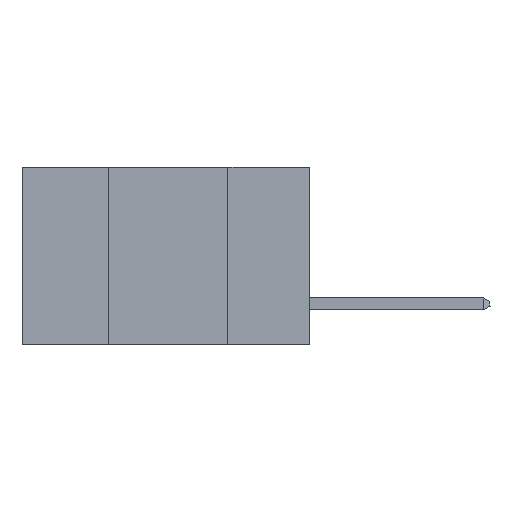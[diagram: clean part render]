
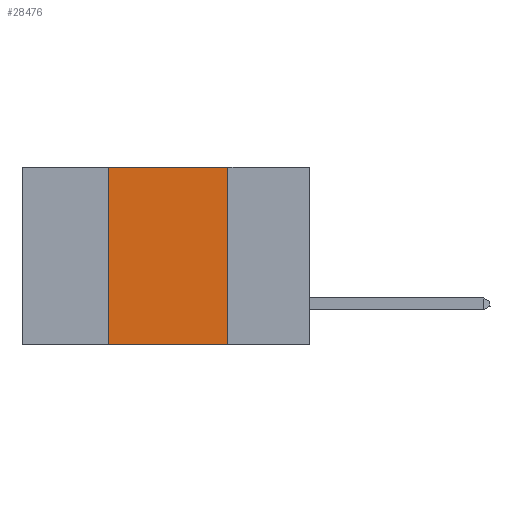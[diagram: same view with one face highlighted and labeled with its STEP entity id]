
A CAD part, left-side view. The second image highlights one B-rep face of the part: STEP entity #28476.
In plain terms, the highlighted planar face has unit normal (-1, 0, 0).
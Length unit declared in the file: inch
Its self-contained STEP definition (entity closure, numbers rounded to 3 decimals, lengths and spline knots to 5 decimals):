
#44 = CARTESIAN_POINT ( 'NONE',  ( 0., 0.6, 0. ) ) ;
#2948 = ORIENTED_EDGE ( 'NONE', *, *, #10224, .F. ) ;
#3013 = VERTEX_POINT ( 'NONE', #19193 ) ;
#5655 = CARTESIAN_POINT ( 'NONE',  ( 0., 0.42, -0.37 ) ) ;
#6412 = ORIENTED_EDGE ( 'NONE', *, *, #18906, .F. ) ;
#6725 = ORIENTED_EDGE ( 'NONE', *, *, #29199, .F. ) ;
#7812 = DIRECTION ( 'NONE',  ( 0., -1., 0. ) ) ;
#8812 = VECTOR ( 'NONE', #7812, 39.37008 ) ;
#9528 = DIRECTION ( 'NONE',  ( 0., 0., -1. ) ) ;
#9575 = DIRECTION ( 'NONE',  ( 1., 0., 0. ) ) ;
#9995 = CARTESIAN_POINT ( 'NONE',  ( 0., 0.6, 0. ) ) ;
#10224 = EDGE_CURVE ( 'NONE', #12231, #34975, #14798, .T. ) ;
#10891 = LINE ( 'NONE', #24702, #37234 ) ;
#12231 = VERTEX_POINT ( 'NONE', #19691 ) ;
#12410 = CARTESIAN_POINT ( 'NONE',  ( 0., 0.17, 0. ) ) ;
#14000 = FACE_OUTER_BOUND ( 'NONE', #26840, .T. ) ;
#14798 = LINE ( 'NONE', #9995, #33801 ) ;
#15305 = DIRECTION ( 'NONE',  ( 0., 0., 1. ) ) ;
#16122 = LINE ( 'NONE', #17218, #8812 ) ;
#17218 = CARTESIAN_POINT ( 'NONE',  ( 0., 0.6, -0.37 ) ) ;
#18651 = AXIS2_PLACEMENT_3D ( 'NONE', #44, #9575, #21847 ) ;
#18726 = PLANE ( 'NONE',  #18651 ) ;
#18906 = EDGE_CURVE ( 'NONE', #25185, #12231, #10891, .T. ) ;
#19193 = CARTESIAN_POINT ( 'NONE',  ( 0., 0.17, -0.37 ) ) ;
#19691 = CARTESIAN_POINT ( 'NONE',  ( 0., 0.42, 0. ) ) ;
#21227 = ORIENTED_EDGE ( 'NONE', *, *, #31779, .T. ) ;
#21847 = DIRECTION ( 'NONE',  ( 0., 0., -1. ) ) ;
#24702 = CARTESIAN_POINT ( 'NONE',  ( 0., 0.42, 0. ) ) ;
#25185 = VERTEX_POINT ( 'NONE', #5655 ) ;
#26840 = EDGE_LOOP ( 'NONE', ( #6725, #2948, #6412, #21227 ) ) ;
#28476 = ADVANCED_FACE ( 'NONE', ( #14000 ), #18726, .F. ) ;
#29199 = EDGE_CURVE ( 'NONE', #34975, #3013, #40308, .T. ) ;
#31779 = EDGE_CURVE ( 'NONE', #25185, #3013, #16122, .T. ) ;
#31996 = VECTOR ( 'NONE', #9528, 39.37008 ) ;
#33801 = VECTOR ( 'NONE', #34414, 39.37008 ) ;
#34414 = DIRECTION ( 'NONE',  ( 0., -1., 0. ) ) ;
#34975 = VERTEX_POINT ( 'NONE', #12410 ) ;
#35296 = CARTESIAN_POINT ( 'NONE',  ( 0., 0.17, 0. ) ) ;
#37234 = VECTOR ( 'NONE', #15305, 39.37008 ) ;
#40308 = LINE ( 'NONE', #35296, #31996 ) ;
